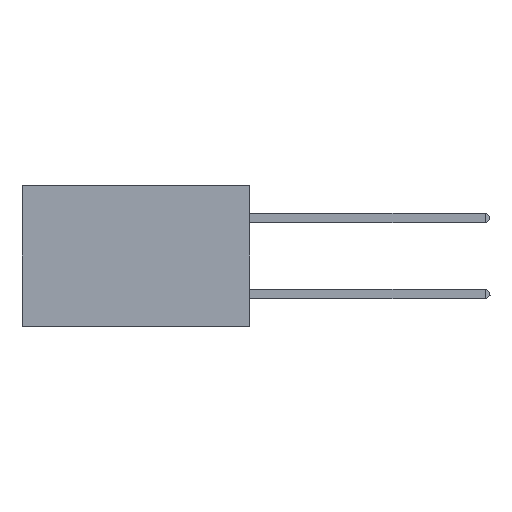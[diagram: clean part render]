
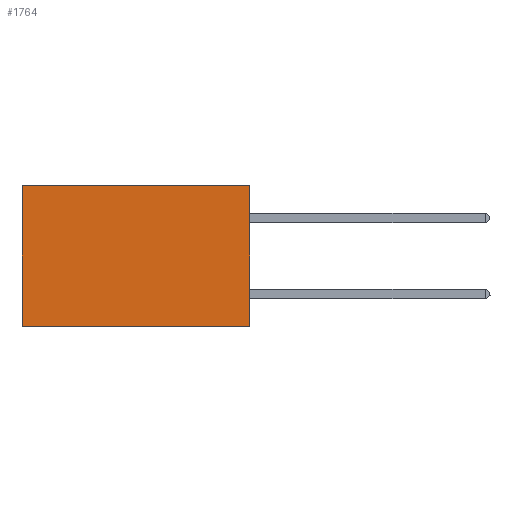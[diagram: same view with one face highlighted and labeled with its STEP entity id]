
A CAD part, left-side view. The second image highlights one B-rep face of the part: STEP entity #1764.
In plain terms, the highlighted planar face has unit normal (-1, 0, 0).
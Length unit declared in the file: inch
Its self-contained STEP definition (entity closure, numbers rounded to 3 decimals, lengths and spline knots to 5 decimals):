
#287 = DIRECTION ( 'NONE',  ( 0., 0., -1. ) ) ;
#603 = DIRECTION ( 'NONE',  ( 0., 0., -1. ) ) ;
#1493 = VERTEX_POINT ( 'NONE', #5136 ) ;
#1612 = CARTESIAN_POINT ( 'NONE',  ( 0.2875, 0., 0. ) ) ;
#1764 = ADVANCED_FACE ( 'NONE', ( #4237 ), #15872, .F. ) ;
#2076 = VERTEX_POINT ( 'NONE', #16145 ) ;
#2230 = LINE ( 'NONE', #1612, #13550 ) ;
#3071 = ORIENTED_EDGE ( 'NONE', *, *, #14136, .T. ) ;
#4155 = ORIENTED_EDGE ( 'NONE', *, *, #10411, .F. ) ;
#4237 = FACE_OUTER_BOUND ( 'NONE', #9006, .T. ) ;
#4356 = EDGE_CURVE ( 'NONE', #8740, #2076, #9137, .T. ) ;
#4484 = CARTESIAN_POINT ( 'NONE',  ( 0.2875, 0., 0. ) ) ;
#4765 = CARTESIAN_POINT ( 'NONE',  ( 0.2875, 0.6, 0. ) ) ;
#5136 = CARTESIAN_POINT ( 'NONE',  ( 0.2875, 0., 0. ) ) ;
#5824 = CARTESIAN_POINT ( 'NONE',  ( 0.2875, 0., -0.37 ) ) ;
#6032 = LINE ( 'NONE', #4765, #16356 ) ;
#6615 = CARTESIAN_POINT ( 'NONE',  ( 0.2875, 0., 0. ) ) ;
#7929 = EDGE_CURVE ( 'NONE', #13975, #2076, #6032, .T. ) ;
#7955 = AXIS2_PLACEMENT_3D ( 'NONE', #4484, #9541, #603 ) ;
#8740 = VERTEX_POINT ( 'NONE', #13381 ) ;
#9006 = EDGE_LOOP ( 'NONE', ( #10854, #12979, #4155, #3071 ) ) ;
#9137 = LINE ( 'NONE', #5824, #10907 ) ;
#9541 = DIRECTION ( 'NONE',  ( 1., 0., 0. ) ) ;
#10281 = VECTOR ( 'NONE', #14261, 39.37008 ) ;
#10411 = EDGE_CURVE ( 'NONE', #1493, #8740, #2230, .T. ) ;
#10854 = ORIENTED_EDGE ( 'NONE', *, *, #7929, .T. ) ;
#10907 = VECTOR ( 'NONE', #16142, 39.37008 ) ;
#11292 = DIRECTION ( 'NONE',  ( 0., 0., -1. ) ) ;
#12058 = LINE ( 'NONE', #6615, #10281 ) ;
#12979 = ORIENTED_EDGE ( 'NONE', *, *, #4356, .F. ) ;
#13381 = CARTESIAN_POINT ( 'NONE',  ( 0.2875, 0., -0.37 ) ) ;
#13550 = VECTOR ( 'NONE', #287, 39.37008 ) ;
#13975 = VERTEX_POINT ( 'NONE', #14931 ) ;
#14136 = EDGE_CURVE ( 'NONE', #1493, #13975, #12058, .T. ) ;
#14261 = DIRECTION ( 'NONE',  ( 0., 1., 0. ) ) ;
#14931 = CARTESIAN_POINT ( 'NONE',  ( 0.2875, 0.6, 0. ) ) ;
#15872 = PLANE ( 'NONE',  #7955 ) ;
#16142 = DIRECTION ( 'NONE',  ( 0., 1., 0. ) ) ;
#16145 = CARTESIAN_POINT ( 'NONE',  ( 0.2875, 0.6, -0.37 ) ) ;
#16356 = VECTOR ( 'NONE', #11292, 39.37008 ) ;
